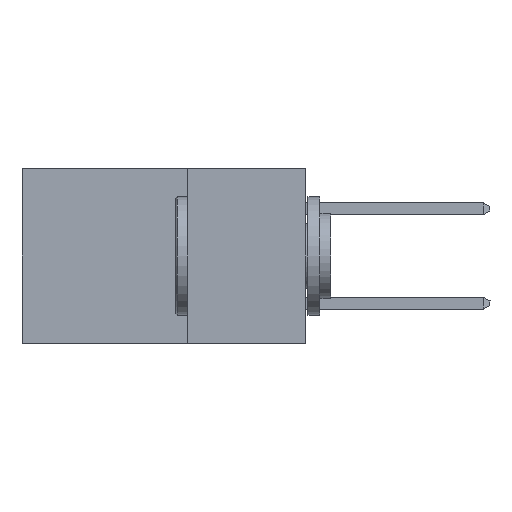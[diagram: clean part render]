
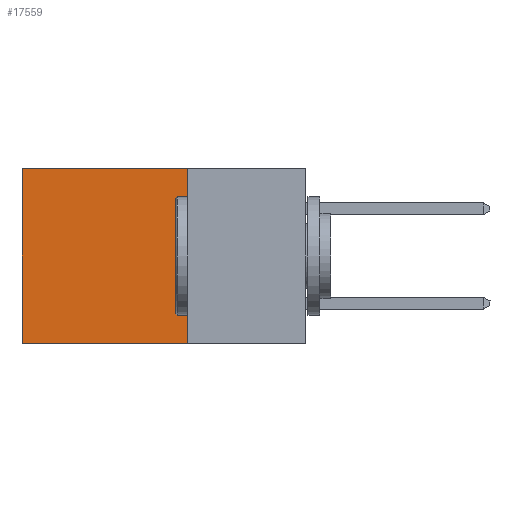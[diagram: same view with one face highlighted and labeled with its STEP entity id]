
A CAD part, left-side view. The second image highlights one B-rep face of the part: STEP entity #17559.
In plain terms, the highlighted planar face has unit normal (-1, 0, 0).
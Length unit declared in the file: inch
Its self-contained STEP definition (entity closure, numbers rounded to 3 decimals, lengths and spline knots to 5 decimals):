
#240 = EDGE_CURVE ( 'NONE', #7259, #14995, #3259, .T. ) ;
#489 = VECTOR ( 'NONE', #3356, 39.37008 ) ;
#868 = ORIENTED_EDGE ( 'NONE', *, *, #5352, .T. ) ;
#1108 = CARTESIAN_POINT ( 'NONE',  ( 0.298, 0.25, 0. ) ) ;
#1525 = EDGE_CURVE ( 'NONE', #3835, #13431, #3004, .T. ) ;
#1629 = CARTESIAN_POINT ( 'NONE',  ( 0.298, 0.25, -0.37 ) ) ;
#2619 = CARTESIAN_POINT ( 'NONE',  ( 0.298, 0.25, -0.37 ) ) ;
#2748 = VECTOR ( 'NONE', #11850, 39.37008 ) ;
#2912 = CARTESIAN_POINT ( 'NONE',  ( 0.298, 0.6, -0.37 ) ) ;
#3004 = LINE ( 'NONE', #1629, #15463 ) ;
#3156 = EDGE_LOOP ( 'NONE', ( #868, #7908, #8276, #16757 ) ) ;
#3169 = FACE_OUTER_BOUND ( 'NONE', #3156, .T. ) ;
#3259 = LINE ( 'NONE', #10524, #7178 ) ;
#3356 = DIRECTION ( 'NONE',  ( 0., 0., -1. ) ) ;
#3539 = CARTESIAN_POINT ( 'NONE',  ( 0.298, 0.25, 0. ) ) ;
#3835 = VERTEX_POINT ( 'NONE', #2619 ) ;
#4375 = DIRECTION ( 'NONE',  ( 0., 1., 0. ) ) ;
#5352 = EDGE_CURVE ( 'NONE', #14995, #13431, #6404, .T. ) ;
#6404 = LINE ( 'NONE', #10367, #2748 ) ;
#7178 = VECTOR ( 'NONE', #10747, 39.37008 ) ;
#7259 = VERTEX_POINT ( 'NONE', #3539 ) ;
#7908 = ORIENTED_EDGE ( 'NONE', *, *, #1525, .F. ) ;
#8018 = DIRECTION ( 'NONE',  ( 1., 0., 0. ) ) ;
#8276 = ORIENTED_EDGE ( 'NONE', *, *, #16122, .F. ) ;
#8402 = LINE ( 'NONE', #10298, #489 ) ;
#10298 = CARTESIAN_POINT ( 'NONE',  ( 0.298, 0.25, 0. ) ) ;
#10367 = CARTESIAN_POINT ( 'NONE',  ( 0.298, 0.6, 0. ) ) ;
#10524 = CARTESIAN_POINT ( 'NONE',  ( 0.298, 0.25, 0. ) ) ;
#10747 = DIRECTION ( 'NONE',  ( 0., 1., 0. ) ) ;
#11850 = DIRECTION ( 'NONE',  ( 0., 0., -1. ) ) ;
#13431 = VERTEX_POINT ( 'NONE', #2912 ) ;
#13455 = PLANE ( 'NONE',  #14222 ) ;
#14222 = AXIS2_PLACEMENT_3D ( 'NONE', #1108, #8018, #16298 ) ;
#14591 = CARTESIAN_POINT ( 'NONE',  ( 0.298, 0.6, 0. ) ) ;
#14995 = VERTEX_POINT ( 'NONE', #14591 ) ;
#15463 = VECTOR ( 'NONE', #4375, 39.37008 ) ;
#16122 = EDGE_CURVE ( 'NONE', #7259, #3835, #8402, .T. ) ;
#16298 = DIRECTION ( 'NONE',  ( 0., 0., -1. ) ) ;
#16757 = ORIENTED_EDGE ( 'NONE', *, *, #240, .T. ) ;
#17559 = ADVANCED_FACE ( 'NONE', ( #3169 ), #13455, .F. ) ;
